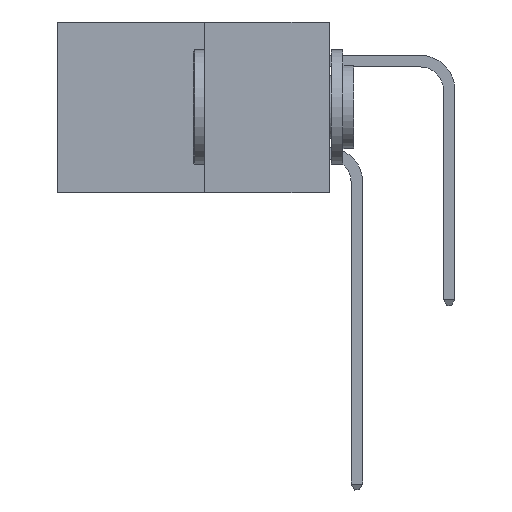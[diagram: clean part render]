
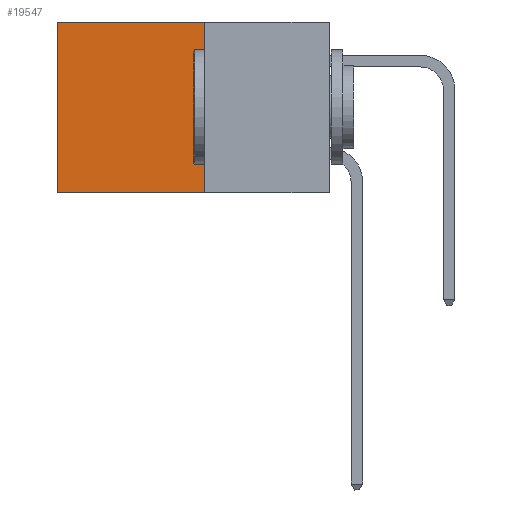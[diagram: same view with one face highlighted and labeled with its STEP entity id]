
A CAD part, left-side view. The second image highlights one B-rep face of the part: STEP entity #19547.
In plain terms, the highlighted planar face has unit normal (-1, 0, 0).
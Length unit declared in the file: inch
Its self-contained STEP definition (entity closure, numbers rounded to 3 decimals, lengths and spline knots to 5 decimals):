
#1402 = ORIENTED_EDGE ( 'NONE', *, *, #8645, .F. ) ;
#1509 = CARTESIAN_POINT ( 'NONE',  ( 0.277, 0.59, 0. ) ) ;
#1995 = DIRECTION ( 'NONE',  ( 0., 1., 0. ) ) ;
#1997 = LINE ( 'NONE', #14363, #8414 ) ;
#2598 = AXIS2_PLACEMENT_3D ( 'NONE', #5676, #8100, #24775 ) ;
#2820 = ORIENTED_EDGE ( 'NONE', *, *, #16331, .T. ) ;
#3232 = PLANE ( 'NONE',  #2598 ) ;
#5070 = FACE_OUTER_BOUND ( 'NONE', #22583, .T. ) ;
#5676 = CARTESIAN_POINT ( 'NONE',  ( 0.277, 0.27, -0.37 ) ) ;
#8100 = DIRECTION ( 'NONE',  ( 1., 0., 0. ) ) ;
#8112 = VECTOR ( 'NONE', #1995, 39.37008 ) ;
#8414 = VECTOR ( 'NONE', #16751, 39.37008 ) ;
#8645 = EDGE_CURVE ( 'NONE', #11544, #26579, #15090, .T. ) ;
#8918 = VERTEX_POINT ( 'NONE', #30498 ) ;
#9104 = ORIENTED_EDGE ( 'NONE', *, *, #13199, .F. ) ;
#9488 = VECTOR ( 'NONE', #27199, 39.37008 ) ;
#10938 = ORIENTED_EDGE ( 'NONE', *, *, #17067, .T. ) ;
#11544 = VERTEX_POINT ( 'NONE', #15528 ) ;
#11675 = CARTESIAN_POINT ( 'NONE',  ( 0.277, 0.59, -0.37 ) ) ;
#12960 = CARTESIAN_POINT ( 'NONE',  ( 0.277, 0.27, -0.37 ) ) ;
#13199 = EDGE_CURVE ( 'NONE', #26579, #8918, #14476, .T. ) ;
#14363 = CARTESIAN_POINT ( 'NONE',  ( 0.277, 0.27, 0. ) ) ;
#14476 = LINE ( 'NONE', #18449, #8112 ) ;
#15090 = LINE ( 'NONE', #12960, #9488 ) ;
#15528 = CARTESIAN_POINT ( 'NONE',  ( 0.277, 0.27, 0. ) ) ;
#15940 = VECTOR ( 'NONE', #30803, 39.37008 ) ;
#16331 = EDGE_CURVE ( 'NONE', #27606, #8918, #22279, .T. ) ;
#16751 = DIRECTION ( 'NONE',  ( 0., 1., 0. ) ) ;
#17067 = EDGE_CURVE ( 'NONE', #11544, #27606, #1997, .T. ) ;
#18449 = CARTESIAN_POINT ( 'NONE',  ( 0.277, 0.27, -0.37 ) ) ;
#19547 = ADVANCED_FACE ( 'NONE', ( #5070 ), #3232, .F. ) ;
#22279 = LINE ( 'NONE', #11675, #15940 ) ;
#22583 = EDGE_LOOP ( 'NONE', ( #2820, #9104, #1402, #10938 ) ) ;
#24775 = DIRECTION ( 'NONE',  ( 0., 0., -1. ) ) ;
#25487 = CARTESIAN_POINT ( 'NONE',  ( 0.277, 0.27, -0.37 ) ) ;
#26579 = VERTEX_POINT ( 'NONE', #25487 ) ;
#27199 = DIRECTION ( 'NONE',  ( 0., 0., -1. ) ) ;
#27606 = VERTEX_POINT ( 'NONE', #1509 ) ;
#30498 = CARTESIAN_POINT ( 'NONE',  ( 0.277, 0.59, -0.37 ) ) ;
#30803 = DIRECTION ( 'NONE',  ( 0., 0., -1. ) ) ;
